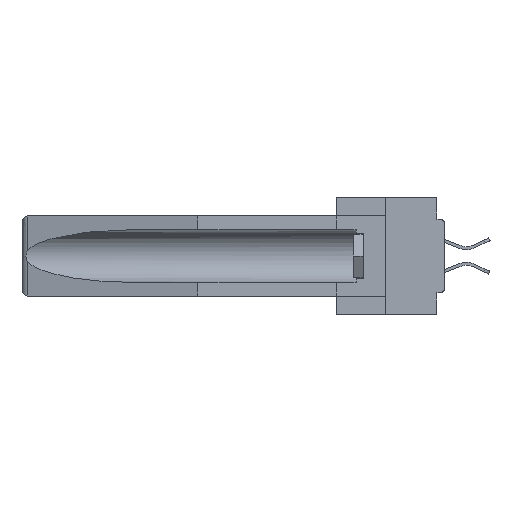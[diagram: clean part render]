
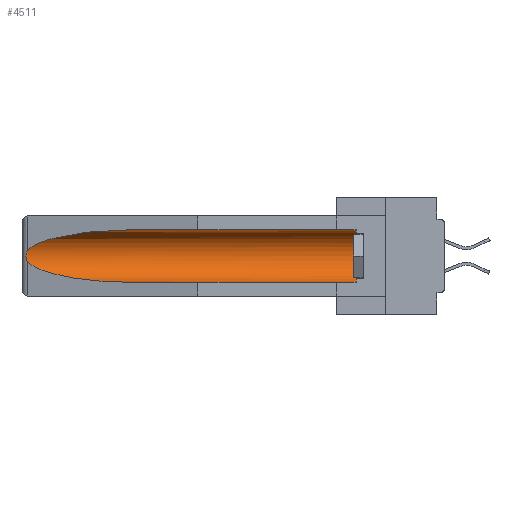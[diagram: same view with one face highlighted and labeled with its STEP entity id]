
A CAD part, left-side view. The second image highlights one B-rep face of the part: STEP entity #4511.
In plain terms, the highlighted cylindrical face has radius 2.857 mm (diameter 5.715 mm), a partial arc.
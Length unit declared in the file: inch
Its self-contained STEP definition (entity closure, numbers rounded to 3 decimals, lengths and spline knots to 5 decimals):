
#1859 = EDGE_CURVE ( 'NONE', #29297, #32016, #20858, .T. ) ;
#3407 = CARTESIAN_POINT ( 'NONE',  ( 0.26537, 1.52718, -0.14972 ) ) ;
#3861 =( BOUNDED_CURVE ( )  B_SPLINE_CURVE ( 3, ( #13240, #24309, #38856, #3407 ),
 .UNSPECIFIED., .F., .T. ) 
 B_SPLINE_CURVE_WITH_KNOTS ( ( 4, 4 ),
 ( 4.71239, 6.08839 ),
 .UNSPECIFIED. ) 
 CURVE ( )  GEOMETRIC_REPRESENTATION_ITEM ( )  RATIONAL_B_SPLINE_CURVE ( ( 1., 0.848, 0.848, 1. ) ) 
 REPRESENTATION_ITEM ( '' )  );
#4305 = DIRECTION ( 'NONE',  ( 0., 0., 1. ) ) ;
#4509 = FACE_OUTER_BOUND ( 'NONE', #13244, .T. ) ;
#4511 = ADVANCED_FACE ( 'NONE', ( #4509 ), #37203, .F. ) ;
#4514 = CARTESIAN_POINT ( 'NONE',  ( 0.2673, 1.53269, -0.17917 ) ) ;
#4874 = ORIENTED_EDGE ( 'NONE', *, *, #27989, .T. ) ;
#4948 = CARTESIAN_POINT ( 'NONE',  ( 0.26537, 1.52718, -0.14972 ) ) ;
#5493 = CARTESIAN_POINT ( 'NONE',  ( 0.155, -0.30754, -0.1715 ) ) ;
#5676 = ORIENTED_EDGE ( 'NONE', *, *, #11293, .T. ) ;
#6031 = ORIENTED_EDGE ( 'NONE', *, *, #39255, .F. ) ;
#7839 = CIRCLE ( 'NONE', #39216, 0.1125 ) ;
#7935 = CARTESIAN_POINT ( 'NONE',  ( 0.2675, 1.53308, -0.16763 ) ) ;
#8176 = DIRECTION ( 'NONE',  ( 0., 1., 0. ) ) ;
#9014 = DIRECTION ( 'NONE',  ( 0., 1., 0. ) ) ;
#10268 = ORIENTED_EDGE ( 'NONE', *, *, #13960, .T. ) ;
#11171 = CARTESIAN_POINT ( 'NONE',  ( 0.26655, 1.53094, -0.18657 ) ) ;
#11293 = EDGE_CURVE ( 'NONE', #32016, #22186, #40003, .T. ) ;
#11806 = CARTESIAN_POINT ( 'NONE',  ( 0.26537, 1.52718, -0.19328 ) ) ;
#11994 = DIRECTION ( 'NONE',  ( 0., 0., 1. ) ) ;
#13240 = CARTESIAN_POINT ( 'NONE',  ( 0.155, 1.07973, -0.059 ) ) ;
#13244 = EDGE_LOOP ( 'NONE', ( #10268, #20883, #5676, #6031, #4874, #17654 ) ) ;
#13960 = EDGE_CURVE ( 'NONE', #36844, #29297, #3861, .T. ) ;
#13978 = DIRECTION ( 'NONE',  ( 0., -1., 0. ) ) ;
#14083 = AXIS2_PLACEMENT_3D ( 'NONE', #5493, #9014, #11994 ) ;
#14639 = CARTESIAN_POINT ( 'NONE',  ( 0.26537, 1.52718, -0.14972 ) ) ;
#15484 = CARTESIAN_POINT ( 'NONE',  ( 0.26597, 1.5296, -0.19026 ) ) ;
#17654 = ORIENTED_EDGE ( 'NONE', *, *, #26077, .T. ) ;
#18121 = CARTESIAN_POINT ( 'NONE',  ( 0.26537, 1.52718, -0.19328 ) ) ;
#18200 = CARTESIAN_POINT ( 'NONE',  ( 0.2675, 1.53308, -0.17534 ) ) ;
#19457 = VERTEX_POINT ( 'NONE', #37496 ) ;
#19693 = CARTESIAN_POINT ( 'NONE',  ( 0.155, 0.126, -0.284 ) ) ;
#20452 = VERTEX_POINT ( 'NONE', #19693 ) ;
#20728 = LINE ( 'NONE', #23030, #33498 ) ;
#20858 = B_SPLINE_CURVE_WITH_KNOTS ( 'NONE', 3,
 ( #4948, #27779, #34324, #37775, #7935, #18200, #4514, #11171, #15484, #38201 ),
 .UNSPECIFIED., .F., .F.,
 ( 4, 2, 2, 2, 4 ),
 ( 0., 0.00029, 0.00058, 0.00087, 0.00117 ),
 .UNSPECIFIED. ) ;
#20883 = ORIENTED_EDGE ( 'NONE', *, *, #1859, .T. ) ;
#21347 = CARTESIAN_POINT ( 'NONE',  ( 0.155, 1.07973, -0.284 ) ) ;
#22186 = VERTEX_POINT ( 'NONE', #21347 ) ;
#23030 = CARTESIAN_POINT ( 'NONE',  ( 0.155, -0.30754, -0.059 ) ) ;
#24309 = CARTESIAN_POINT ( 'NONE',  ( 0.21114, 1.30732, -0.059 ) ) ;
#26077 = EDGE_CURVE ( 'NONE', #19457, #36844, #20728, .T. ) ;
#27779 = CARTESIAN_POINT ( 'NONE',  ( 0.26597, 1.52961, -0.15275 ) ) ;
#27986 = CARTESIAN_POINT ( 'NONE',  ( 0.155, 1.07973, -0.059 ) ) ;
#27989 = EDGE_CURVE ( 'NONE', #20452, #19457, #7839, .T. ) ;
#28551 = CARTESIAN_POINT ( 'NONE',  ( 0.25451, 1.48313, -0.24835 ) ) ;
#29297 = VERTEX_POINT ( 'NONE', #14639 ) ;
#29352 = DIRECTION ( 'NONE',  ( 0., 1., 0. ) ) ;
#31560 = CARTESIAN_POINT ( 'NONE',  ( 0.21114, 1.30732, -0.284 ) ) ;
#31847 = CARTESIAN_POINT ( 'NONE',  ( 0.155, 1.07973, -0.284 ) ) ;
#32016 = VERTEX_POINT ( 'NONE', #11806 ) ;
#33498 = VECTOR ( 'NONE', #29352, 39.37008 ) ;
#33537 = CARTESIAN_POINT ( 'NONE',  ( 0.155, 0.126, -0.1715 ) ) ;
#34324 = CARTESIAN_POINT ( 'NONE',  ( 0.26654, 1.53092, -0.15636 ) ) ;
#34563 = CARTESIAN_POINT ( 'NONE',  ( 0.155, -0.30754, -0.284 ) ) ;
#35452 = VECTOR ( 'NONE', #8176, 39.37008 ) ;
#36844 = VERTEX_POINT ( 'NONE', #27986 ) ;
#37203 = CYLINDRICAL_SURFACE ( 'NONE', #14083, 0.1125 ) ;
#37496 = CARTESIAN_POINT ( 'NONE',  ( 0.155, 0.126, -0.059 ) ) ;
#37775 = CARTESIAN_POINT ( 'NONE',  ( 0.2673, 1.5327, -0.16383 ) ) ;
#38201 = CARTESIAN_POINT ( 'NONE',  ( 0.26537, 1.52718, -0.19328 ) ) ;
#38856 = CARTESIAN_POINT ( 'NONE',  ( 0.25451, 1.48313, -0.09465 ) ) ;
#39216 = AXIS2_PLACEMENT_3D ( 'NONE', #33537, #13978, #4305 ) ;
#39255 = EDGE_CURVE ( 'NONE', #20452, #22186, #40598, .T. ) ;
#40003 =( BOUNDED_CURVE ( )  B_SPLINE_CURVE ( 3, ( #18121, #28551, #31560, #31847 ),
 .UNSPECIFIED., .F., .T. ) 
 B_SPLINE_CURVE_WITH_KNOTS ( ( 4, 4 ),
 ( 0.1948, 1.5708 ),
 .UNSPECIFIED. ) 
 CURVE ( )  GEOMETRIC_REPRESENTATION_ITEM ( )  RATIONAL_B_SPLINE_CURVE ( ( 1., 0.848, 0.848, 1. ) ) 
 REPRESENTATION_ITEM ( '' )  );
#40598 = LINE ( 'NONE', #34563, #35452 ) ;
